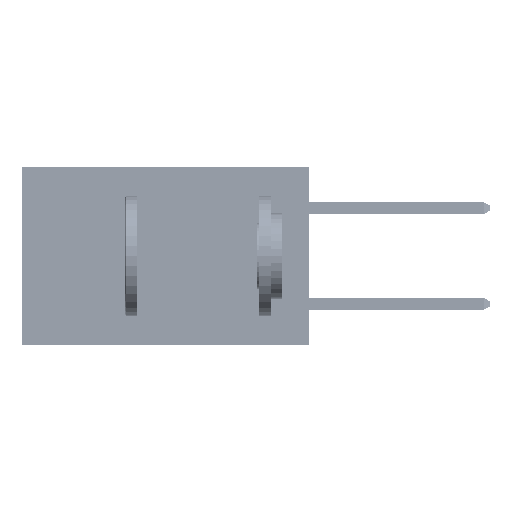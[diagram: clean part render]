
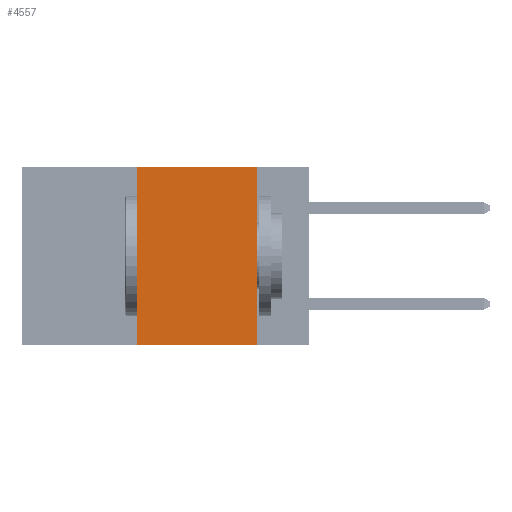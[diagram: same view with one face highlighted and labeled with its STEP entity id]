
A CAD part, left-side view. The second image highlights one B-rep face of the part: STEP entity #4557.
In plain terms, the highlighted planar face has unit normal (-1, 0, 0).
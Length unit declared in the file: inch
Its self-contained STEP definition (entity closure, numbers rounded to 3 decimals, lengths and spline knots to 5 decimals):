
#3101 = EDGE_CURVE ( 'NONE', #36752, #6738, #38914, .T. ) ;
#3131 = ORIENTED_EDGE ( 'NONE', *, *, #16429, .F. ) ;
#3816 = CARTESIAN_POINT ( 'NONE',  ( 0., 0.6, 0. ) ) ;
#4210 = CARTESIAN_POINT ( 'NONE',  ( 0., 0.6, 0. ) ) ;
#4557 = ADVANCED_FACE ( 'NONE', ( #6796 ), #22712, .F. ) ;
#4804 = LINE ( 'NONE', #27349, #15832 ) ;
#5929 = CARTESIAN_POINT ( 'NONE',  ( 0., 0.11, 0. ) ) ;
#6738 = VERTEX_POINT ( 'NONE', #17822 ) ;
#6796 = FACE_OUTER_BOUND ( 'NONE', #47639, .T. ) ;
#9546 = CARTESIAN_POINT ( 'NONE',  ( 0., 0.36, -0.37 ) ) ;
#9688 = CARTESIAN_POINT ( 'NONE',  ( 0., 0.11, 0. ) ) ;
#12237 = LINE ( 'NONE', #5929, #33171 ) ;
#13841 = VECTOR ( 'NONE', #33522, 39.37008 ) ;
#15393 = DIRECTION ( 'NONE',  ( 1., 0., 0. ) ) ;
#15595 = ORIENTED_EDGE ( 'NONE', *, *, #24752, .T. ) ;
#15832 = VECTOR ( 'NONE', #46466, 39.37008 ) ;
#16429 = EDGE_CURVE ( 'NONE', #32357, #38428, #12237, .T. ) ;
#17822 = CARTESIAN_POINT ( 'NONE',  ( 0., 0.36, 0. ) ) ;
#22712 = PLANE ( 'NONE',  #41672 ) ;
#23508 = CARTESIAN_POINT ( 'NONE',  ( 0., 0.11, -0.37 ) ) ;
#23723 = DIRECTION ( 'NONE',  ( 0., 0., 1. ) ) ;
#24752 = EDGE_CURVE ( 'NONE', #36752, #38428, #4804, .T. ) ;
#26774 = DIRECTION ( 'NONE',  ( 0., 0., -1. ) ) ;
#27349 = CARTESIAN_POINT ( 'NONE',  ( 0., 0.6, -0.37 ) ) ;
#30705 = LINE ( 'NONE', #3816, #13841 ) ;
#31133 = ORIENTED_EDGE ( 'NONE', *, *, #3101, .F. ) ;
#32228 = DIRECTION ( 'NONE',  ( 0., 0., -1. ) ) ;
#32357 = VERTEX_POINT ( 'NONE', #9688 ) ;
#33171 = VECTOR ( 'NONE', #32228, 39.37008 ) ;
#33522 = DIRECTION ( 'NONE',  ( 0., -1., 0. ) ) ;
#33866 = EDGE_CURVE ( 'NONE', #6738, #32357, #30705, .T. ) ;
#36752 = VERTEX_POINT ( 'NONE', #9546 ) ;
#38428 = VERTEX_POINT ( 'NONE', #23508 ) ;
#38914 = LINE ( 'NONE', #38980, #45883 ) ;
#38980 = CARTESIAN_POINT ( 'NONE',  ( 0., 0.36, 0. ) ) ;
#41672 = AXIS2_PLACEMENT_3D ( 'NONE', #4210, #15393, #26774 ) ;
#44336 = ORIENTED_EDGE ( 'NONE', *, *, #33866, .F. ) ;
#45883 = VECTOR ( 'NONE', #23723, 39.37008 ) ;
#46466 = DIRECTION ( 'NONE',  ( 0., -1., 0. ) ) ;
#47639 = EDGE_LOOP ( 'NONE', ( #3131, #44336, #31133, #15595 ) ) ;
